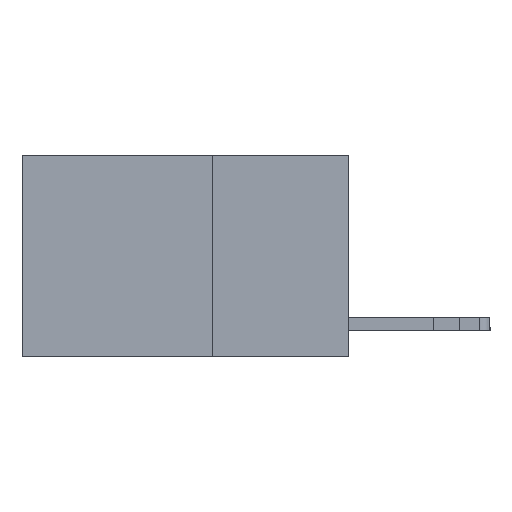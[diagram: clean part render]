
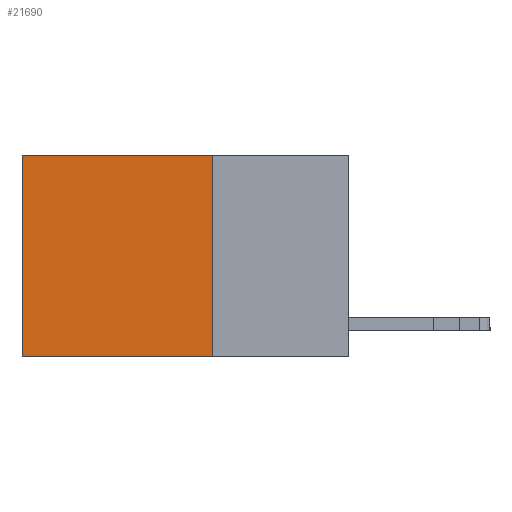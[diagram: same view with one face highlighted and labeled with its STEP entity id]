
A CAD part, left-side view. The second image highlights one B-rep face of the part: STEP entity #21690.
In plain terms, the highlighted planar face has unit normal (-1, 0, 0).
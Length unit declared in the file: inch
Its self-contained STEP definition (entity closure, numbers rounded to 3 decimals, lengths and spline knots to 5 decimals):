
#69 = EDGE_CURVE ( 'NONE', #9607, #19762, #16539, .T. ) ;
#285 = CARTESIAN_POINT ( 'NONE',  ( 0.2625, 0.25, -0.37 ) ) ;
#2870 = EDGE_CURVE ( 'NONE', #12998, #19762, #21209, .T. ) ;
#3650 = CARTESIAN_POINT ( 'NONE',  ( 0.2625, 0.25, -0.37 ) ) ;
#3879 = CARTESIAN_POINT ( 'NONE',  ( 0.2625, 0.25, 0. ) ) ;
#4708 = ORIENTED_EDGE ( 'NONE', *, *, #2870, .F. ) ;
#4804 = CARTESIAN_POINT ( 'NONE',  ( 0.2625, 0.25, 0. ) ) ;
#4812 = CARTESIAN_POINT ( 'NONE',  ( 0.2625, 0.6, 0. ) ) ;
#4924 = PLANE ( 'NONE',  #22042 ) ;
#5936 = DIRECTION ( 'NONE',  ( 0., 1., 0. ) ) ;
#6746 = DIRECTION ( 'NONE',  ( 1., 0., 0. ) ) ;
#7864 = VECTOR ( 'NONE', #24429, 39.37008 ) ;
#8908 = CARTESIAN_POINT ( 'NONE',  ( 0.2625, 0.25, 0. ) ) ;
#9607 = VERTEX_POINT ( 'NONE', #11988 ) ;
#10619 = ORIENTED_EDGE ( 'NONE', *, *, #69, .T. ) ;
#11397 = CARTESIAN_POINT ( 'NONE',  ( 0.2625, 0.6, -0.37 ) ) ;
#11644 = DIRECTION ( 'NONE',  ( 0., 1., 0. ) ) ;
#11988 = CARTESIAN_POINT ( 'NONE',  ( 0.2625, 0.6, 0. ) ) ;
#12781 = DIRECTION ( 'NONE',  ( 0., 0., -1. ) ) ;
#12998 = VERTEX_POINT ( 'NONE', #285 ) ;
#14042 = ORIENTED_EDGE ( 'NONE', *, *, #15086, .T. ) ;
#15086 = EDGE_CURVE ( 'NONE', #23383, #9607, #19984, .T. ) ;
#15479 = LINE ( 'NONE', #3879, #19862 ) ;
#16539 = LINE ( 'NONE', #4812, #7864 ) ;
#17386 = EDGE_LOOP ( 'NONE', ( #10619, #4708, #19202, #14042 ) ) ;
#18041 = CARTESIAN_POINT ( 'NONE',  ( 0.2625, 0.25, 0. ) ) ;
#19202 = ORIENTED_EDGE ( 'NONE', *, *, #25458, .F. ) ;
#19762 = VERTEX_POINT ( 'NONE', #11397 ) ;
#19862 = VECTOR ( 'NONE', #25440, 39.37008 ) ;
#19908 = VECTOR ( 'NONE', #11644, 39.37008 ) ;
#19984 = LINE ( 'NONE', #18041, #20348 ) ;
#20348 = VECTOR ( 'NONE', #5936, 39.37008 ) ;
#21209 = LINE ( 'NONE', #3650, #19908 ) ;
#21690 = ADVANCED_FACE ( 'NONE', ( #24416 ), #4924, .F. ) ;
#22042 = AXIS2_PLACEMENT_3D ( 'NONE', #4804, #6746, #12781 ) ;
#23383 = VERTEX_POINT ( 'NONE', #8908 ) ;
#24416 = FACE_OUTER_BOUND ( 'NONE', #17386, .T. ) ;
#24429 = DIRECTION ( 'NONE',  ( 0., 0., -1. ) ) ;
#25440 = DIRECTION ( 'NONE',  ( 0., 0., -1. ) ) ;
#25458 = EDGE_CURVE ( 'NONE', #23383, #12998, #15479, .T. ) ;
